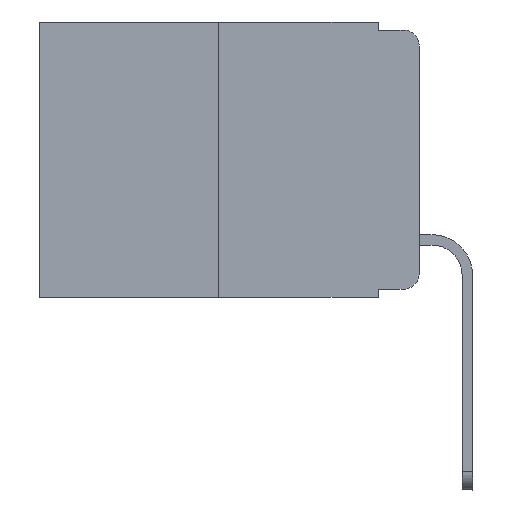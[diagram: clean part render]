
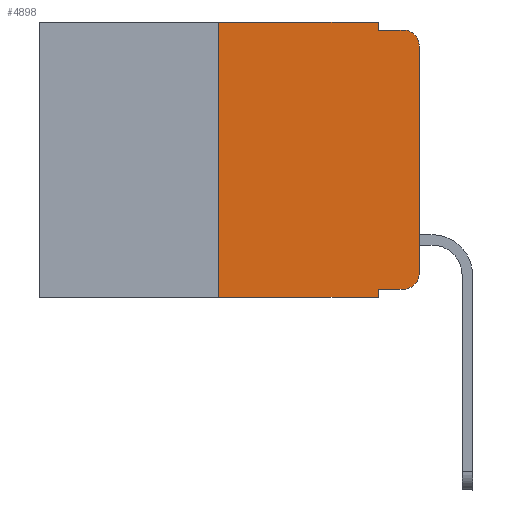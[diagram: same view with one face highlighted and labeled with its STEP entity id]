
A CAD part, left-side view. The second image highlights one B-rep face of the part: STEP entity #4898.
In plain terms, the highlighted planar face has unit normal (-1, 0, 0).
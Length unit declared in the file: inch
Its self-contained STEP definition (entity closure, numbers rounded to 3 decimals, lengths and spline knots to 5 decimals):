
#310 = AXIS2_PLACEMENT_3D ( 'NONE', #7451, #3415, #6592 ) ;
#403 = VECTOR ( 'NONE', #3507, 39.37008 ) ;
#425 = EDGE_CURVE ( 'NONE', #4892, #6782, #1889, .T. ) ;
#433 = VERTEX_POINT ( 'NONE', #1180 ) ;
#614 = CARTESIAN_POINT ( 'NONE',  ( 0., 0.25, -0.343 ) ) ;
#1068 = CARTESIAN_POINT ( 'NONE',  ( 0., 0.051, 0. ) ) ;
#1180 = CARTESIAN_POINT ( 'NONE',  ( 0., 0.02, -0.333 ) ) ;
#1258 = ORIENTED_EDGE ( 'NONE', *, *, #5742, .F. ) ;
#1361 = CARTESIAN_POINT ( 'NONE',  ( 0., 0., 0. ) ) ;
#1430 = LINE ( 'NONE', #6785, #4553 ) ;
#1439 = EDGE_CURVE ( 'NONE', #1512, #7946, #7474, .T. ) ;
#1460 = CARTESIAN_POINT ( 'NONE',  ( 0., 0., -0.03 ) ) ;
#1512 = VERTEX_POINT ( 'NONE', #7787 ) ;
#1578 = VECTOR ( 'NONE', #8348, 39.37008 ) ;
#1863 = DIRECTION ( 'NONE',  ( -1., 0., 0. ) ) ;
#1889 = LINE ( 'NONE', #3360, #403 ) ;
#2115 = LINE ( 'NONE', #3478, #6384 ) ;
#2287 = LINE ( 'NONE', #4616, #4998 ) ;
#2355 = DIRECTION ( 'NONE',  ( 0., 0., -1. ) ) ;
#2458 = EDGE_CURVE ( 'NONE', #7980, #4892, #2287, .T. ) ;
#2551 = EDGE_CURVE ( 'NONE', #433, #1512, #4674, .T. ) ;
#2731 = DIRECTION ( 'NONE',  ( 0., 0., -1. ) ) ;
#2742 = CARTESIAN_POINT ( 'NONE',  ( 0., 0.051, 0. ) ) ;
#3051 = EDGE_CURVE ( 'NONE', #4997, #433, #3665, .T. ) ;
#3225 = CARTESIAN_POINT ( 'NONE',  ( 0., 0.25, 0. ) ) ;
#3345 = VERTEX_POINT ( 'NONE', #8787 ) ;
#3360 = CARTESIAN_POINT ( 'NONE',  ( 0., 0.051, -0.01 ) ) ;
#3415 = DIRECTION ( 'NONE',  ( 1., 0., 0. ) ) ;
#3478 = CARTESIAN_POINT ( 'NONE',  ( 0., 0.473, 0. ) ) ;
#3507 = DIRECTION ( 'NONE',  ( 0., -1., 0. ) ) ;
#3588 = LINE ( 'NONE', #1068, #3785 ) ;
#3608 = CARTESIAN_POINT ( 'NONE',  ( 0., 0.051, -0.01 ) ) ;
#3665 = LINE ( 'NONE', #7514, #10073 ) ;
#3707 = EDGE_CURVE ( 'NONE', #6330, #3345, #1430, .T. ) ;
#3785 = VECTOR ( 'NONE', #8253, 39.37008 ) ;
#3827 = CIRCLE ( 'NONE', #5802, 0.02 ) ;
#3932 = LINE ( 'NONE', #3225, #4692 ) ;
#4286 = ORIENTED_EDGE ( 'NONE', *, *, #2458, .F. ) ;
#4553 = VECTOR ( 'NONE', #8417, 39.37008 ) ;
#4616 = CARTESIAN_POINT ( 'NONE',  ( 0., 0.051, 0. ) ) ;
#4674 = CIRCLE ( 'NONE', #4829, 0.02 ) ;
#4692 = VECTOR ( 'NONE', #7080, 39.37008 ) ;
#4829 = AXIS2_PLACEMENT_3D ( 'NONE', #5748, #1863, #2731 ) ;
#4892 = VERTEX_POINT ( 'NONE', #3608 ) ;
#4898 = ADVANCED_FACE ( 'NONE', ( #5146 ), #7400, .F. ) ;
#4997 = VERTEX_POINT ( 'NONE', #7661 ) ;
#4998 = VECTOR ( 'NONE', #7750, 39.37008 ) ;
#5086 = ORIENTED_EDGE ( 'NONE', *, *, #3051, .T. ) ;
#5146 = FACE_OUTER_BOUND ( 'NONE', #8711, .T. ) ;
#5659 = ORIENTED_EDGE ( 'NONE', *, *, #8981, .T. ) ;
#5742 = EDGE_CURVE ( 'NONE', #8060, #7980, #2115, .T. ) ;
#5748 = CARTESIAN_POINT ( 'NONE',  ( 0., 0.02, -0.313 ) ) ;
#5802 = AXIS2_PLACEMENT_3D ( 'NONE', #6281, #9346, #2355 ) ;
#6281 = CARTESIAN_POINT ( 'NONE',  ( 0., 0.02, -0.03 ) ) ;
#6330 = VERTEX_POINT ( 'NONE', #614 ) ;
#6384 = VECTOR ( 'NONE', #6607, 39.37008 ) ;
#6522 = ORIENTED_EDGE ( 'NONE', *, *, #425, .F. ) ;
#6592 = DIRECTION ( 'NONE',  ( 0., 0., -1. ) ) ;
#6607 = DIRECTION ( 'NONE',  ( 0., -1., 0. ) ) ;
#6703 = DIRECTION ( 'NONE',  ( 0., -1., 0. ) ) ;
#6782 = VERTEX_POINT ( 'NONE', #9181 ) ;
#6785 = CARTESIAN_POINT ( 'NONE',  ( 0., 0.473, -0.343 ) ) ;
#6984 = EDGE_CURVE ( 'NONE', #4997, #3345, #3588, .T. ) ;
#7080 = DIRECTION ( 'NONE',  ( 0., 0., 1. ) ) ;
#7400 = PLANE ( 'NONE',  #310 ) ;
#7414 = ORIENTED_EDGE ( 'NONE', *, *, #6984, .F. ) ;
#7451 = CARTESIAN_POINT ( 'NONE',  ( 0., 0.473, 0. ) ) ;
#7474 = LINE ( 'NONE', #1361, #1578 ) ;
#7514 = CARTESIAN_POINT ( 'NONE',  ( 0., 0.051, -0.333 ) ) ;
#7661 = CARTESIAN_POINT ( 'NONE',  ( 0., 0.051, -0.333 ) ) ;
#7750 = DIRECTION ( 'NONE',  ( 0., 0., -1. ) ) ;
#7787 = CARTESIAN_POINT ( 'NONE',  ( 0., 0., -0.313 ) ) ;
#7946 = VERTEX_POINT ( 'NONE', #1460 ) ;
#7980 = VERTEX_POINT ( 'NONE', #2742 ) ;
#8003 = ORIENTED_EDGE ( 'NONE', *, *, #2551, .T. ) ;
#8060 = VERTEX_POINT ( 'NONE', #8658 ) ;
#8253 = DIRECTION ( 'NONE',  ( 0., 0., -1. ) ) ;
#8348 = DIRECTION ( 'NONE',  ( 0., 0., 1. ) ) ;
#8417 = DIRECTION ( 'NONE',  ( 0., -1., 0. ) ) ;
#8658 = CARTESIAN_POINT ( 'NONE',  ( 0., 0.25, 0. ) ) ;
#8711 = EDGE_LOOP ( 'NONE', ( #9650, #5659, #6522, #4286, #1258, #9836, #9005, #7414, #5086, #8003 ) ) ;
#8787 = CARTESIAN_POINT ( 'NONE',  ( 0., 0.051, -0.343 ) ) ;
#8981 = EDGE_CURVE ( 'NONE', #7946, #6782, #3827, .T. ) ;
#9005 = ORIENTED_EDGE ( 'NONE', *, *, #3707, .T. ) ;
#9181 = CARTESIAN_POINT ( 'NONE',  ( 0., 0.02, -0.01 ) ) ;
#9346 = DIRECTION ( 'NONE',  ( -1., 0., 0. ) ) ;
#9650 = ORIENTED_EDGE ( 'NONE', *, *, #1439, .T. ) ;
#9836 = ORIENTED_EDGE ( 'NONE', *, *, #9848, .F. ) ;
#9848 = EDGE_CURVE ( 'NONE', #6330, #8060, #3932, .T. ) ;
#10073 = VECTOR ( 'NONE', #6703, 39.37008 ) ;
